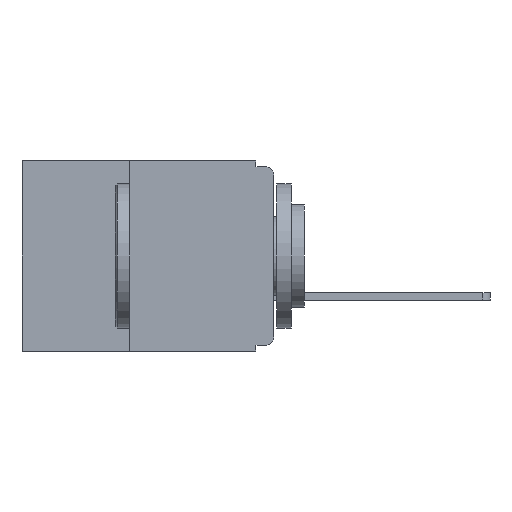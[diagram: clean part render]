
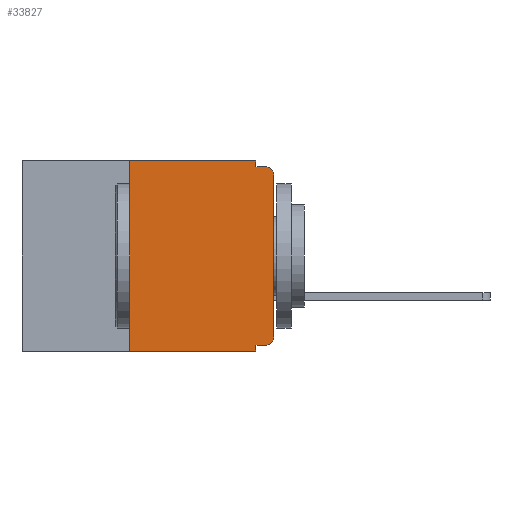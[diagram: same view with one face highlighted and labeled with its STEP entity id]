
A CAD part, left-side view. The second image highlights one B-rep face of the part: STEP entity #33827.
In plain terms, the highlighted planar face has unit normal (-1, 0, 0).
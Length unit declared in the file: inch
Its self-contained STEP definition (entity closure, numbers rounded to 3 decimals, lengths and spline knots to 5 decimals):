
#62 = ORIENTED_EDGE ( 'NONE', *, *, #28687, .F. ) ;
#108 = CARTESIAN_POINT ( 'NONE',  ( 0., 0.031, 0. ) ) ;
#923 = EDGE_CURVE ( 'NONE', #19172, #25381, #28616, .T. ) ;
#1170 = EDGE_CURVE ( 'NONE', #32931, #32670, #19630, .T. ) ;
#1403 = VERTEX_POINT ( 'NONE', #25500 ) ;
#1605 = CARTESIAN_POINT ( 'NONE',  ( 0., 0., -0.01 ) ) ;
#2028 = ORIENTED_EDGE ( 'NONE', *, *, #2189, .T. ) ;
#2041 = ORIENTED_EDGE ( 'NONE', *, *, #20427, .F. ) ;
#2157 = CARTESIAN_POINT ( 'NONE',  ( 0., 0.031, -0.01 ) ) ;
#2189 = EDGE_CURVE ( 'NONE', #19520, #32931, #30942, .T. ) ;
#2704 = CARTESIAN_POINT ( 'NONE',  ( 0., 0.031, -0.33 ) ) ;
#3226 = LINE ( 'NONE', #16971, #29387 ) ;
#3323 = AXIS2_PLACEMENT_3D ( 'NONE', #9560, #27760, #12186 ) ;
#3417 = AXIS2_PLACEMENT_3D ( 'NONE', #23781, #23762, #23537 ) ;
#3609 = ORIENTED_EDGE ( 'NONE', *, *, #5051, .F. ) ;
#3984 = DIRECTION ( 'NONE',  ( 0., 0., -1. ) ) ;
#4524 = ORIENTED_EDGE ( 'NONE', *, *, #12574, .T. ) ;
#4712 = CARTESIAN_POINT ( 'NONE',  ( 0., 0.015, -0.01 ) ) ;
#5051 = EDGE_CURVE ( 'NONE', #6218, #11252, #18961, .T. ) ;
#5331 = ORIENTED_EDGE ( 'NONE', *, *, #20875, .F. ) ;
#5685 = ORIENTED_EDGE ( 'NONE', *, *, #19879, .T. ) ;
#5930 = DIRECTION ( 'NONE',  ( 1., 0., 0. ) ) ;
#6218 = VERTEX_POINT ( 'NONE', #108 ) ;
#6574 = DIRECTION ( 'NONE',  ( 0., 1., 0. ) ) ;
#7499 = LINE ( 'NONE', #29275, #8331 ) ;
#7542 = ORIENTED_EDGE ( 'NONE', *, *, #923, .F. ) ;
#7721 = ORIENTED_EDGE ( 'NONE', *, *, #9260, .F. ) ;
#7823 = VERTEX_POINT ( 'NONE', #4712 ) ;
#7833 = ORIENTED_EDGE ( 'NONE', *, *, #1170, .T. ) ;
#7855 = VECTOR ( 'NONE', #3984, 39.37008 ) ;
#7967 = LINE ( 'NONE', #1605, #22629 ) ;
#8331 = VECTOR ( 'NONE', #11068, 39.37008 ) ;
#8362 = VECTOR ( 'NONE', #27375, 39.37008 ) ;
#9179 = CARTESIAN_POINT ( 'NONE',  ( 0., 0.437, 0. ) ) ;
#9260 = EDGE_CURVE ( 'NONE', #11252, #7823, #7967, .T. ) ;
#9560 = CARTESIAN_POINT ( 'NONE',  ( 0., 0.015, -0.025 ) ) ;
#11068 = DIRECTION ( 'NONE',  ( 0., 0., 1. ) ) ;
#11252 = VERTEX_POINT ( 'NONE', #2157 ) ;
#11716 = CARTESIAN_POINT ( 'NONE',  ( 0., 0., 0. ) ) ;
#12186 = DIRECTION ( 'NONE',  ( 0., 0., -1. ) ) ;
#12469 = CIRCLE ( 'NONE', #3323, 0.015 ) ;
#12549 = CARTESIAN_POINT ( 'NONE',  ( 0., 0.437, -0.33 ) ) ;
#12574 = EDGE_CURVE ( 'NONE', #1403, #25381, #26070, .T. ) ;
#12662 = CARTESIAN_POINT ( 'NONE',  ( 0., 0.031, -0.32 ) ) ;
#12717 = VECTOR ( 'NONE', #19811, 39.37008 ) ;
#15813 = AXIS2_PLACEMENT_3D ( 'NONE', #16331, #5930, #24174 ) ;
#16331 = CARTESIAN_POINT ( 'NONE',  ( 0., 0.437, 0. ) ) ;
#16346 = EDGE_LOOP ( 'NONE', ( #7833, #5685, #7721, #3609, #2041, #5331, #4524, #7542, #62, #2028 ) ) ;
#16971 = CARTESIAN_POINT ( 'NONE',  ( 0., 0., -0.32 ) ) ;
#17402 = FACE_OUTER_BOUND ( 'NONE', #16346, .T. ) ;
#18245 = CARTESIAN_POINT ( 'NONE',  ( 0., 0.031, 0. ) ) ;
#18351 = DIRECTION ( 'NONE',  ( 0., 0., -1. ) ) ;
#18961 = LINE ( 'NONE', #18245, #31964 ) ;
#19172 = VERTEX_POINT ( 'NONE', #12662 ) ;
#19520 = VERTEX_POINT ( 'NONE', #21968 ) ;
#19630 = LINE ( 'NONE', #11716, #12717 ) ;
#19811 = DIRECTION ( 'NONE',  ( 0., 0., 1. ) ) ;
#19879 = EDGE_CURVE ( 'NONE', #32670, #7823, #12469, .T. ) ;
#19961 = DIRECTION ( 'NONE',  ( 0., -1., 0. ) ) ;
#20427 = EDGE_CURVE ( 'NONE', #31512, #6218, #29110, .T. ) ;
#20875 = EDGE_CURVE ( 'NONE', #1403, #31512, #7499, .T. ) ;
#21578 = PLANE ( 'NONE',  #15813 ) ;
#21939 = CARTESIAN_POINT ( 'NONE',  ( 0., 0.25, 0. ) ) ;
#21968 = CARTESIAN_POINT ( 'NONE',  ( 0., 0.015, -0.32 ) ) ;
#22629 = VECTOR ( 'NONE', #19961, 39.37008 ) ;
#23537 = DIRECTION ( 'NONE',  ( 0., 0., -1. ) ) ;
#23563 = CARTESIAN_POINT ( 'NONE',  ( 0., 0.031, -0.33 ) ) ;
#23762 = DIRECTION ( 'NONE',  ( -1., 0., 0. ) ) ;
#23781 = CARTESIAN_POINT ( 'NONE',  ( 0., 0.015, -0.305 ) ) ;
#24174 = DIRECTION ( 'NONE',  ( 0., 0., -1. ) ) ;
#25381 = VERTEX_POINT ( 'NONE', #2704 ) ;
#25500 = CARTESIAN_POINT ( 'NONE',  ( 0., 0.25, -0.33 ) ) ;
#26070 = LINE ( 'NONE', #12549, #32160 ) ;
#27375 = DIRECTION ( 'NONE',  ( 0., -1., 0. ) ) ;
#27760 = DIRECTION ( 'NONE',  ( -1., 0., 0. ) ) ;
#28228 = CARTESIAN_POINT ( 'NONE',  ( 0., 0., -0.305 ) ) ;
#28616 = LINE ( 'NONE', #23563, #7855 ) ;
#28687 = EDGE_CURVE ( 'NONE', #19520, #19172, #3226, .T. ) ;
#29110 = LINE ( 'NONE', #9179, #8362 ) ;
#29275 = CARTESIAN_POINT ( 'NONE',  ( 0., 0.25, -0.33 ) ) ;
#29387 = VECTOR ( 'NONE', #6574, 39.37008 ) ;
#30942 = CIRCLE ( 'NONE', #3417, 0.015 ) ;
#31512 = VERTEX_POINT ( 'NONE', #21939 ) ;
#31853 = CARTESIAN_POINT ( 'NONE',  ( 0., 0., -0.025 ) ) ;
#31964 = VECTOR ( 'NONE', #18351, 39.37008 ) ;
#32160 = VECTOR ( 'NONE', #33333, 39.37008 ) ;
#32670 = VERTEX_POINT ( 'NONE', #31853 ) ;
#32931 = VERTEX_POINT ( 'NONE', #28228 ) ;
#33333 = DIRECTION ( 'NONE',  ( 0., -1., 0. ) ) ;
#33827 = ADVANCED_FACE ( 'NONE', ( #17402 ), #21578, .F. ) ;
